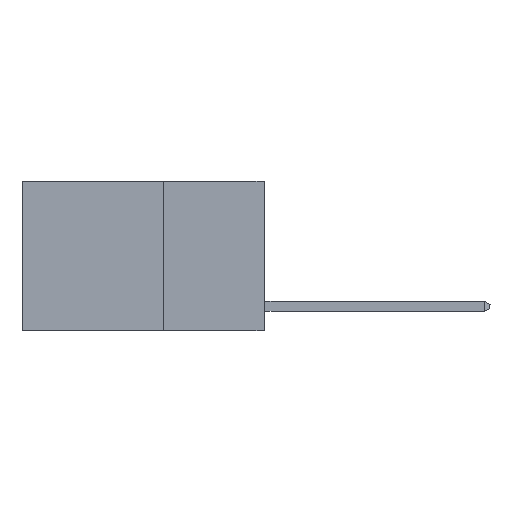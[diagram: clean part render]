
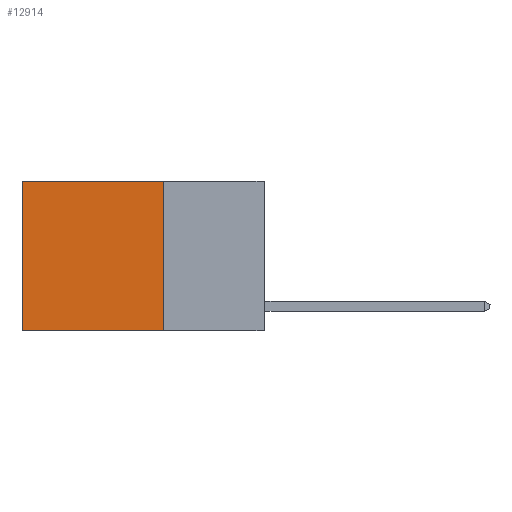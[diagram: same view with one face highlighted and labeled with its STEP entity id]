
A CAD part, left-side view. The second image highlights one B-rep face of the part: STEP entity #12914.
In plain terms, the highlighted planar face has unit normal (-1, 0, 0).
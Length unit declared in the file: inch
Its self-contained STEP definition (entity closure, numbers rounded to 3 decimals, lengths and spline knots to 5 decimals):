
#43 = CARTESIAN_POINT ( 'NONE',  ( 0.2625, 0.25, -0.37 ) ) ;
#183 = VECTOR ( 'NONE', #4027, 39.37008 ) ;
#530 = DIRECTION ( 'NONE',  ( 0., 0., -1. ) ) ;
#871 = DIRECTION ( 'NONE',  ( 0., 0., -1. ) ) ;
#1722 = AXIS2_PLACEMENT_3D ( 'NONE', #1826, #3835, #871 ) ;
#1826 = CARTESIAN_POINT ( 'NONE',  ( 0.2625, 0.25, 0. ) ) ;
#2499 = EDGE_CURVE ( 'NONE', #3290, #8453, #8439, .T. ) ;
#2522 = DIRECTION ( 'NONE',  ( 0., 0., -1. ) ) ;
#3098 = EDGE_CURVE ( 'NONE', #3290, #3357, #12007, .T. ) ;
#3290 = VERTEX_POINT ( 'NONE', #9900 ) ;
#3357 = VERTEX_POINT ( 'NONE', #7008 ) ;
#3807 = ORIENTED_EDGE ( 'NONE', *, *, #2499, .T. ) ;
#3835 = DIRECTION ( 'NONE',  ( 1., 0., 0. ) ) ;
#4027 = DIRECTION ( 'NONE',  ( 0., 1., 0. ) ) ;
#4139 = LINE ( 'NONE', #4541, #4286 ) ;
#4286 = VECTOR ( 'NONE', #530, 39.37008 ) ;
#4399 = CARTESIAN_POINT ( 'NONE',  ( 0.2625, 0.6, 0. ) ) ;
#4541 = CARTESIAN_POINT ( 'NONE',  ( 0.2625, 0.6, 0. ) ) ;
#4839 = EDGE_CURVE ( 'NONE', #8453, #7180, #4139, .T. ) ;
#5713 = EDGE_CURVE ( 'NONE', #3357, #7180, #5992, .T. ) ;
#5992 = LINE ( 'NONE', #43, #183 ) ;
#6831 = PLANE ( 'NONE',  #1722 ) ;
#7008 = CARTESIAN_POINT ( 'NONE',  ( 0.2625, 0.25, -0.37 ) ) ;
#7180 = VERTEX_POINT ( 'NONE', #7258 ) ;
#7258 = CARTESIAN_POINT ( 'NONE',  ( 0.2625, 0.6, -0.37 ) ) ;
#7508 = DIRECTION ( 'NONE',  ( 0., 1., 0. ) ) ;
#8439 = LINE ( 'NONE', #12662, #8750 ) ;
#8453 = VERTEX_POINT ( 'NONE', #4399 ) ;
#8750 = VECTOR ( 'NONE', #7508, 39.37008 ) ;
#9515 = ORIENTED_EDGE ( 'NONE', *, *, #3098, .F. ) ;
#9626 = ORIENTED_EDGE ( 'NONE', *, *, #4839, .T. ) ;
#9900 = CARTESIAN_POINT ( 'NONE',  ( 0.2625, 0.25, 0. ) ) ;
#10121 = FACE_OUTER_BOUND ( 'NONE', #11038, .T. ) ;
#10534 = ORIENTED_EDGE ( 'NONE', *, *, #5713, .F. ) ;
#10615 = VECTOR ( 'NONE', #2522, 39.37008 ) ;
#11038 = EDGE_LOOP ( 'NONE', ( #9626, #10534, #9515, #3807 ) ) ;
#11610 = CARTESIAN_POINT ( 'NONE',  ( 0.2625, 0.25, 0. ) ) ;
#12007 = LINE ( 'NONE', #11610, #10615 ) ;
#12662 = CARTESIAN_POINT ( 'NONE',  ( 0.2625, 0.25, 0. ) ) ;
#12914 = ADVANCED_FACE ( 'NONE', ( #10121 ), #6831, .F. ) ;
